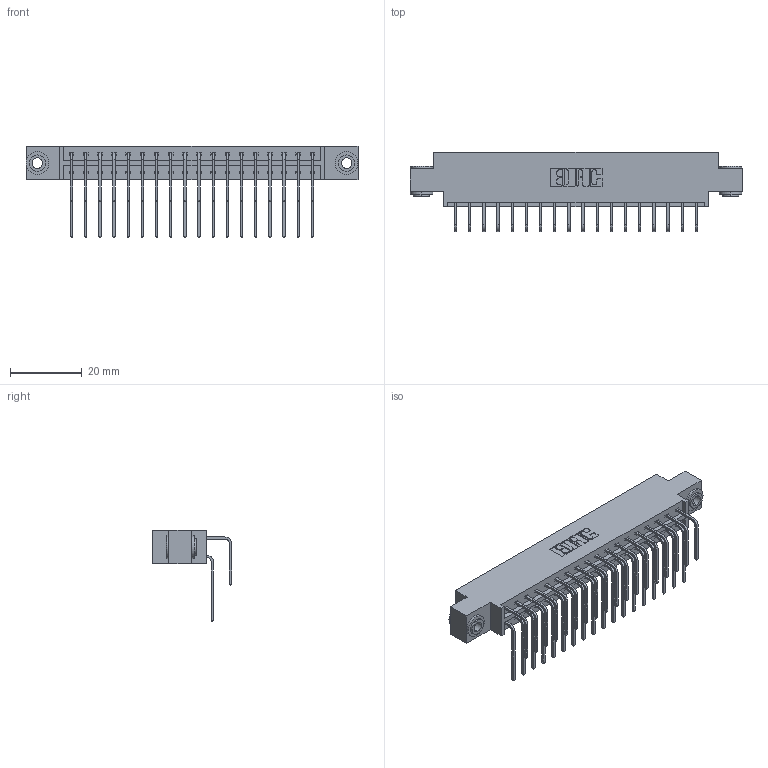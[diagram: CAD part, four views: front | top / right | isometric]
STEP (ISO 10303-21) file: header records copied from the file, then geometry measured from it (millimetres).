
FILE_DESCRIPTION (( 'STEP AP203' ), '1' );
FILE_NAME ('333-036-558-803.STEP', '2018-08-03T01:48:39', ( '' ), ( '' ), 'SwSTEP 2.0', 'SolidWorks 2016', '' );
FILE_SCHEMA (( 'CONFIG_CONTROL_DESIGN' ));
Length unit declared in the file: inch
Products named in the file (5): 333 Part_Offset - .156 Dia - TH; 345-292-001_558 559 Tail - 1; 345-292-001_558 Tail - 2; 345-250-002_345-250-002-102; 333-036-558-803
Assembly tree (39 placements, depth 2):
  333-036-558-803
    333 Part_Offset - .156 Dia - TH
    345-292-001_558 559 Tail - 1  x18
    345-292-001_558 Tail - 2  x18
    345-250-002_345-250-002-102  x2
Bounding box: 92.86 x 22.17 x 25.53 mm (x, y, z)
Volume: 9255.6 mm3; surface area: 12160.6 mm2
Topology: 39 solids, 39 shells, 2100 faces, 6195 edges, 4078 vertices
Faces by surface type: plane 1452, cylinder 640, cone 8
Entity records: 17250 total; most frequent: CARTESIAN_POINT 2916, ORIENTED_EDGE 2794, DIRECTION 2547, EDGE_CURVE 1397, LINE 1205, VECTOR 1205, VERTEX_POINT 926, AXIS2_PLACEMENT_3D 671
